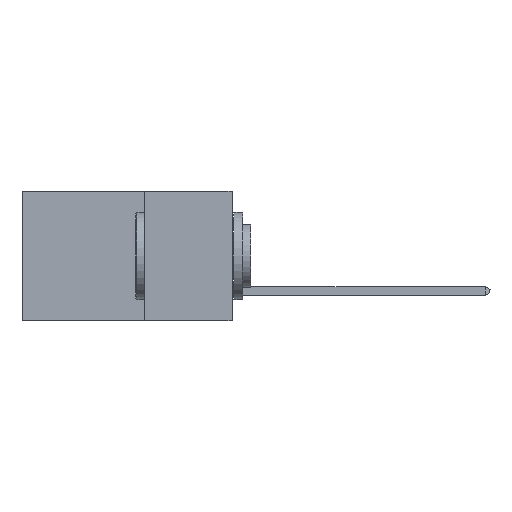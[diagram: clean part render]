
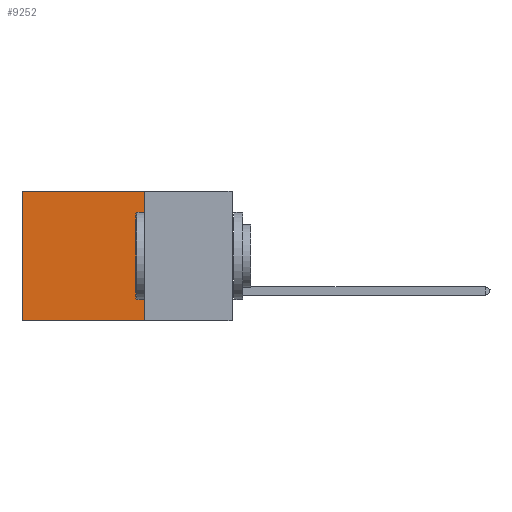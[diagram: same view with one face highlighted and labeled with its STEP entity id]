
A CAD part, left-side view. The second image highlights one B-rep face of the part: STEP entity #9252.
In plain terms, the highlighted planar face has unit normal (-1, 0, 0).
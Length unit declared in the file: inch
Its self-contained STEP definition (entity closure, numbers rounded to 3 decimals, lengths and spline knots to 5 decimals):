
#1305 = CARTESIAN_POINT ( 'NONE',  ( 0.2875, 0.25, 0. ) ) ;
#1994 = DIRECTION ( 'NONE',  ( 0., 1., 0. ) ) ;
#2022 = CARTESIAN_POINT ( 'NONE',  ( 0.2875, 0.25, 0. ) ) ;
#3763 = LINE ( 'NONE', #16165, #8196 ) ;
#4755 = ORIENTED_EDGE ( 'NONE', *, *, #42993, .T. ) ;
#4902 = DIRECTION ( 'NONE',  ( 0., 0., -1. ) ) ;
#6240 = ORIENTED_EDGE ( 'NONE', *, *, #26638, .T. ) ;
#6638 = VERTEX_POINT ( 'NONE', #1305 ) ;
#7664 = VERTEX_POINT ( 'NONE', #10071 ) ;
#8196 = VECTOR ( 'NONE', #1994, 39.37008 ) ;
#9140 = DIRECTION ( 'NONE',  ( 1., 0., 0. ) ) ;
#9252 = ADVANCED_FACE ( 'NONE', ( #42674 ), #9295, .F. ) ;
#9295 = PLANE ( 'NONE',  #40266 ) ;
#10071 = CARTESIAN_POINT ( 'NONE',  ( 0.2875, 0.6, 0. ) ) ;
#12891 = DIRECTION ( 'NONE',  ( 0., 0., -1. ) ) ;
#15189 = CARTESIAN_POINT ( 'NONE',  ( 0.2875, 0.25, 0. ) ) ;
#15683 = LINE ( 'NONE', #30068, #31118 ) ;
#16165 = CARTESIAN_POINT ( 'NONE',  ( 0.2875, 0.25, 0. ) ) ;
#16311 = ORIENTED_EDGE ( 'NONE', *, *, #36547, .F. ) ;
#16342 = DIRECTION ( 'NONE',  ( 0., 0., -1. ) ) ;
#17412 = CARTESIAN_POINT ( 'NONE',  ( 0.2875, 0.25, -0.37 ) ) ;
#22766 = ORIENTED_EDGE ( 'NONE', *, *, #24047, .F. ) ;
#24047 = EDGE_CURVE ( 'NONE', #39308, #37281, #15683, .T. ) ;
#26638 = EDGE_CURVE ( 'NONE', #6638, #7664, #3763, .T. ) ;
#29928 = LINE ( 'NONE', #34322, #33261 ) ;
#30068 = CARTESIAN_POINT ( 'NONE',  ( 0.2875, 0.25, -0.37 ) ) ;
#31118 = VECTOR ( 'NONE', #43967, 39.37008 ) ;
#33261 = VECTOR ( 'NONE', #12891, 39.37008 ) ;
#33677 = CARTESIAN_POINT ( 'NONE',  ( 0.2875, 0.6, -0.37 ) ) ;
#34322 = CARTESIAN_POINT ( 'NONE',  ( 0.2875, 0.6, 0. ) ) ;
#36547 = EDGE_CURVE ( 'NONE', #6638, #39308, #38312, .T. ) ;
#36967 = EDGE_LOOP ( 'NONE', ( #4755, #22766, #16311, #6240 ) ) ;
#37281 = VERTEX_POINT ( 'NONE', #33677 ) ;
#38312 = LINE ( 'NONE', #15189, #39418 ) ;
#39308 = VERTEX_POINT ( 'NONE', #17412 ) ;
#39418 = VECTOR ( 'NONE', #4902, 39.37008 ) ;
#40266 = AXIS2_PLACEMENT_3D ( 'NONE', #2022, #9140, #16342 ) ;
#42674 = FACE_OUTER_BOUND ( 'NONE', #36967, .T. ) ;
#42993 = EDGE_CURVE ( 'NONE', #7664, #37281, #29928, .T. ) ;
#43967 = DIRECTION ( 'NONE',  ( 0., 1., 0. ) ) ;
